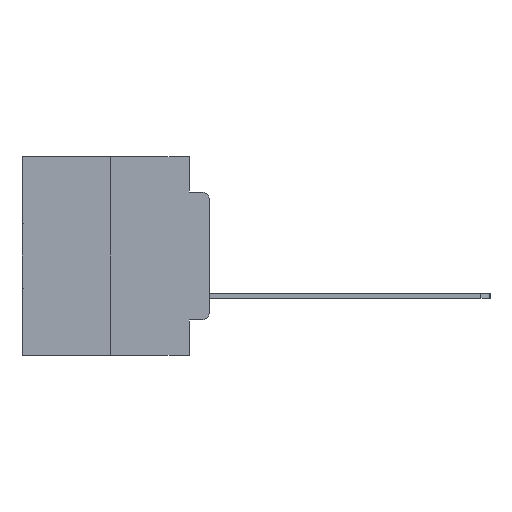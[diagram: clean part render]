
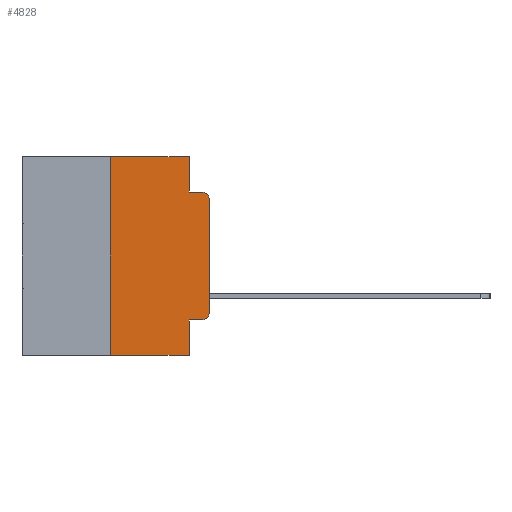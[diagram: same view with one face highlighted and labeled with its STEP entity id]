
A CAD part, left-side view. The second image highlights one B-rep face of the part: STEP entity #4828.
In plain terms, the highlighted planar face has unit normal (-1, 0, 0).
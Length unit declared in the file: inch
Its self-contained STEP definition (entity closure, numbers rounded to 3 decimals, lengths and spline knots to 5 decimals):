
#411 = VERTEX_POINT ( 'NONE', #4035 ) ;
#544 = ORIENTED_EDGE ( 'NONE', *, *, #2392, .F. ) ;
#1145 = CIRCLE ( 'NONE', #15216, 0.02 ) ;
#1151 = VECTOR ( 'NONE', #6971, 39.37008 ) ;
#1590 = LINE ( 'NONE', #12800, #7389 ) ;
#1742 = CARTESIAN_POINT ( 'NONE',  ( 0., 0.473, 0. ) ) ;
#2392 = EDGE_CURVE ( 'NONE', #26115, #19742, #16333, .T. ) ;
#2679 = DIRECTION ( 'NONE',  ( 0., 0., -1. ) ) ;
#2713 = CARTESIAN_POINT ( 'NONE',  ( 0., 0.25, 0. ) ) ;
#2919 = CARTESIAN_POINT ( 'NONE',  ( 0., 0.02, -0.0885 ) ) ;
#3202 = LINE ( 'NONE', #27085, #25193 ) ;
#3321 = FACE_OUTER_BOUND ( 'NONE', #18371, .T. ) ;
#4035 = CARTESIAN_POINT ( 'NONE',  ( 0., 0., -0.3915 ) ) ;
#4392 = VECTOR ( 'NONE', #23541, 39.37008 ) ;
#4490 = CARTESIAN_POINT ( 'NONE',  ( 0., 0., -0.1085 ) ) ;
#4783 = CARTESIAN_POINT ( 'NONE',  ( 0., 0.473, -0.5 ) ) ;
#4828 = ADVANCED_FACE ( 'NONE', ( #3321 ), #5425, .F. ) ;
#5035 = CARTESIAN_POINT ( 'NONE',  ( 0., 0.25, 0. ) ) ;
#5100 = EDGE_CURVE ( 'NONE', #9196, #22558, #1590, .T. ) ;
#5168 = CARTESIAN_POINT ( 'NONE',  ( 0., 0.02, -0.1085 ) ) ;
#5216 = DIRECTION ( 'NONE',  ( 0., 0., -1. ) ) ;
#5339 = DIRECTION ( 'NONE',  ( 1., 0., 0. ) ) ;
#5425 = PLANE ( 'NONE',  #25010 ) ;
#5606 = CARTESIAN_POINT ( 'NONE',  ( 0., 0.051, 0. ) ) ;
#6328 = VERTEX_POINT ( 'NONE', #24302 ) ;
#6540 = EDGE_CURVE ( 'NONE', #9196, #13598, #3202, .T. ) ;
#6971 = DIRECTION ( 'NONE',  ( 0., -1., 0. ) ) ;
#6984 = CARTESIAN_POINT ( 'NONE',  ( 0., 0.473, 0. ) ) ;
#7066 = CARTESIAN_POINT ( 'NONE',  ( 0., 0.051, 0. ) ) ;
#7149 = CARTESIAN_POINT ( 'NONE',  ( 0., 0.051, -0.4115 ) ) ;
#7365 = DIRECTION ( 'NONE',  ( 0., 0., -1. ) ) ;
#7389 = VECTOR ( 'NONE', #12891, 39.37008 ) ;
#7744 = CIRCLE ( 'NONE', #25682, 0.02 ) ;
#7818 = CARTESIAN_POINT ( 'NONE',  ( 0., 0., 0. ) ) ;
#7849 = VERTEX_POINT ( 'NONE', #4490 ) ;
#8014 = EDGE_CURVE ( 'NONE', #6328, #26115, #18952, .T. ) ;
#8428 = ORIENTED_EDGE ( 'NONE', *, *, #6540, .F. ) ;
#9196 = VERTEX_POINT ( 'NONE', #7149 ) ;
#9646 = DIRECTION ( 'NONE',  ( 0., -1., 0. ) ) ;
#10790 = ORIENTED_EDGE ( 'NONE', *, *, #12356, .F. ) ;
#10928 = EDGE_CURVE ( 'NONE', #19742, #23102, #20575, .T. ) ;
#12079 = DIRECTION ( 'NONE',  ( 0., 0., 1. ) ) ;
#12128 = ORIENTED_EDGE ( 'NONE', *, *, #8014, .F. ) ;
#12152 = CARTESIAN_POINT ( 'NONE',  ( 0., 0.02, -0.3915 ) ) ;
#12356 = EDGE_CURVE ( 'NONE', #23102, #14431, #21465, .T. ) ;
#12800 = CARTESIAN_POINT ( 'NONE',  ( 0., 0.051, -0.4115 ) ) ;
#12891 = DIRECTION ( 'NONE',  ( 0., -1., 0. ) ) ;
#13313 = VECTOR ( 'NONE', #26284, 39.37008 ) ;
#13598 = VERTEX_POINT ( 'NONE', #27541 ) ;
#13814 = EDGE_CURVE ( 'NONE', #7849, #14431, #7744, .T. ) ;
#14279 = VECTOR ( 'NONE', #2679, 39.37008 ) ;
#14304 = DIRECTION ( 'NONE',  ( 0., 0., -1. ) ) ;
#14431 = VERTEX_POINT ( 'NONE', #2919 ) ;
#15136 = ORIENTED_EDGE ( 'NONE', *, *, #15237, .T. ) ;
#15216 = AXIS2_PLACEMENT_3D ( 'NONE', #12152, #26840, #14304 ) ;
#15237 = EDGE_CURVE ( 'NONE', #411, #7849, #26173, .T. ) ;
#15490 = ORIENTED_EDGE ( 'NONE', *, *, #5100, .T. ) ;
#15730 = VECTOR ( 'NONE', #12079, 39.37008 ) ;
#16333 = LINE ( 'NONE', #1742, #21283 ) ;
#18350 = LINE ( 'NONE', #4783, #1151 ) ;
#18371 = EDGE_LOOP ( 'NONE', ( #15136, #26908, #10790, #22709, #544, #12128, #18451, #8428, #15490, #26600 ) ) ;
#18451 = ORIENTED_EDGE ( 'NONE', *, *, #21234, .T. ) ;
#18822 = DIRECTION ( 'NONE',  ( 0., 0., -1. ) ) ;
#18952 = LINE ( 'NONE', #5035, #13313 ) ;
#19742 = VERTEX_POINT ( 'NONE', #5606 ) ;
#20183 = DIRECTION ( 'NONE',  ( -1., 0., 0. ) ) ;
#20575 = LINE ( 'NONE', #7066, #14279 ) ;
#21234 = EDGE_CURVE ( 'NONE', #6328, #13598, #18350, .T. ) ;
#21283 = VECTOR ( 'NONE', #9646, 39.37008 ) ;
#21432 = CARTESIAN_POINT ( 'NONE',  ( 0., 0.051, -0.0885 ) ) ;
#21465 = LINE ( 'NONE', #21432, #4392 ) ;
#22558 = VERTEX_POINT ( 'NONE', #22664 ) ;
#22664 = CARTESIAN_POINT ( 'NONE',  ( 0., 0.02, -0.4115 ) ) ;
#22709 = ORIENTED_EDGE ( 'NONE', *, *, #10928, .F. ) ;
#23102 = VERTEX_POINT ( 'NONE', #26523 ) ;
#23541 = DIRECTION ( 'NONE',  ( 0., -1., 0. ) ) ;
#24302 = CARTESIAN_POINT ( 'NONE',  ( 0., 0.25, -0.5 ) ) ;
#25010 = AXIS2_PLACEMENT_3D ( 'NONE', #6984, #5339, #5216 ) ;
#25193 = VECTOR ( 'NONE', #18822, 39.37008 ) ;
#25682 = AXIS2_PLACEMENT_3D ( 'NONE', #5168, #20183, #7365 ) ;
#26115 = VERTEX_POINT ( 'NONE', #2713 ) ;
#26173 = LINE ( 'NONE', #7818, #15730 ) ;
#26284 = DIRECTION ( 'NONE',  ( 0., 0., 1. ) ) ;
#26523 = CARTESIAN_POINT ( 'NONE',  ( 0., 0.051, -0.0885 ) ) ;
#26600 = ORIENTED_EDGE ( 'NONE', *, *, #26955, .T. ) ;
#26840 = DIRECTION ( 'NONE',  ( -1., 0., 0. ) ) ;
#26908 = ORIENTED_EDGE ( 'NONE', *, *, #13814, .T. ) ;
#26955 = EDGE_CURVE ( 'NONE', #22558, #411, #1145, .T. ) ;
#27085 = CARTESIAN_POINT ( 'NONE',  ( 0., 0.051, 0. ) ) ;
#27541 = CARTESIAN_POINT ( 'NONE',  ( 0., 0.051, -0.5 ) ) ;
